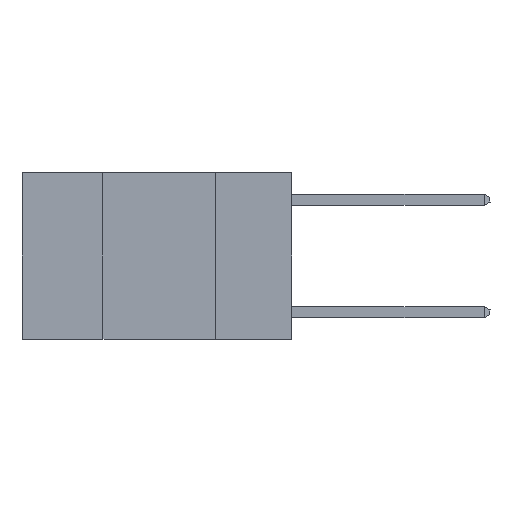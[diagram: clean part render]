
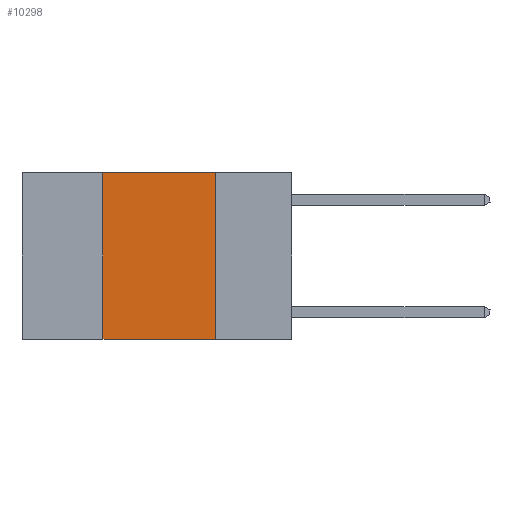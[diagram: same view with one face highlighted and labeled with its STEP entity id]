
A CAD part, left-side view. The second image highlights one B-rep face of the part: STEP entity #10298.
In plain terms, the highlighted planar face has unit normal (-1, 0, 0).
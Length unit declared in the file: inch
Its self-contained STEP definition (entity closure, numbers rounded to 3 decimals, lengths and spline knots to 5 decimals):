
#2159 = EDGE_LOOP ( 'NONE', ( #20606, #3615, #12630, #27780 ) ) ;
#3122 = LINE ( 'NONE', #11540, #9681 ) ;
#3239 = DIRECTION ( 'NONE',  ( 0., 0., -1. ) ) ;
#3615 = ORIENTED_EDGE ( 'NONE', *, *, #23403, .F. ) ;
#4175 = EDGE_CURVE ( 'NONE', #11394, #18756, #10028, .T. ) ;
#4886 = CARTESIAN_POINT ( 'NONE',  ( 0., 0.42, -0.37 ) ) ;
#5433 = CARTESIAN_POINT ( 'NONE',  ( 0., 0.6, 0. ) ) ;
#5556 = EDGE_CURVE ( 'NONE', #11394, #27724, #6895, .T. ) ;
#6808 = VERTEX_POINT ( 'NONE', #8518 ) ;
#6895 = LINE ( 'NONE', #18010, #15646 ) ;
#7579 = DIRECTION ( 'NONE',  ( 1., 0., 0. ) ) ;
#8518 = CARTESIAN_POINT ( 'NONE',  ( 0., 0.17, 0. ) ) ;
#8538 = DIRECTION ( 'NONE',  ( 0., 0., 1. ) ) ;
#9312 = AXIS2_PLACEMENT_3D ( 'NONE', #5433, #7579, #3239 ) ;
#9681 = VECTOR ( 'NONE', #14411, 39.37008 ) ;
#9902 = PLANE ( 'NONE',  #9312 ) ;
#10028 = LINE ( 'NONE', #24114, #23937 ) ;
#10298 = ADVANCED_FACE ( 'NONE', ( #20703 ), #9902, .F. ) ;
#11394 = VERTEX_POINT ( 'NONE', #4886 ) ;
#11540 = CARTESIAN_POINT ( 'NONE',  ( 0., 0.6, 0. ) ) ;
#12630 = ORIENTED_EDGE ( 'NONE', *, *, #4175, .F. ) ;
#12714 = CARTESIAN_POINT ( 'NONE',  ( 0., 0.17, 0. ) ) ;
#14411 = DIRECTION ( 'NONE',  ( 0., -1., 0. ) ) ;
#15646 = VECTOR ( 'NONE', #20173, 39.37008 ) ;
#18010 = CARTESIAN_POINT ( 'NONE',  ( 0., 0.6, -0.37 ) ) ;
#18756 = VERTEX_POINT ( 'NONE', #18934 ) ;
#18934 = CARTESIAN_POINT ( 'NONE',  ( 0., 0.42, 0. ) ) ;
#20173 = DIRECTION ( 'NONE',  ( 0., -1., 0. ) ) ;
#20606 = ORIENTED_EDGE ( 'NONE', *, *, #27201, .F. ) ;
#20703 = FACE_OUTER_BOUND ( 'NONE', #2159, .T. ) ;
#23210 = DIRECTION ( 'NONE',  ( 0., 0., -1. ) ) ;
#23403 = EDGE_CURVE ( 'NONE', #18756, #6808, #3122, .T. ) ;
#23937 = VECTOR ( 'NONE', #8538, 39.37008 ) ;
#24114 = CARTESIAN_POINT ( 'NONE',  ( 0., 0.42, 0. ) ) ;
#24517 = VECTOR ( 'NONE', #23210, 39.37008 ) ;
#25255 = LINE ( 'NONE', #12714, #24517 ) ;
#27201 = EDGE_CURVE ( 'NONE', #6808, #27724, #25255, .T. ) ;
#27724 = VERTEX_POINT ( 'NONE', #28096 ) ;
#27780 = ORIENTED_EDGE ( 'NONE', *, *, #5556, .T. ) ;
#28096 = CARTESIAN_POINT ( 'NONE',  ( 0., 0.17, -0.37 ) ) ;
